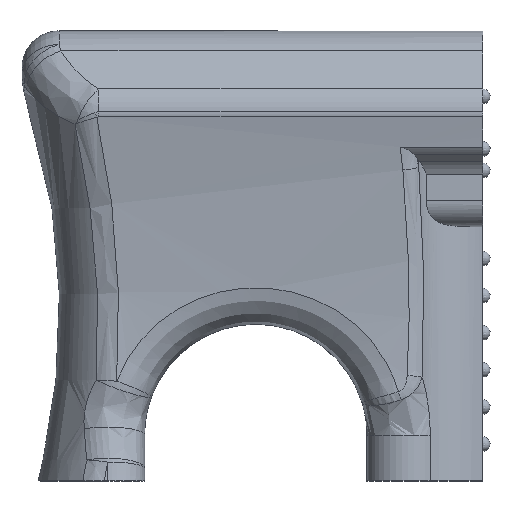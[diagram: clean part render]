
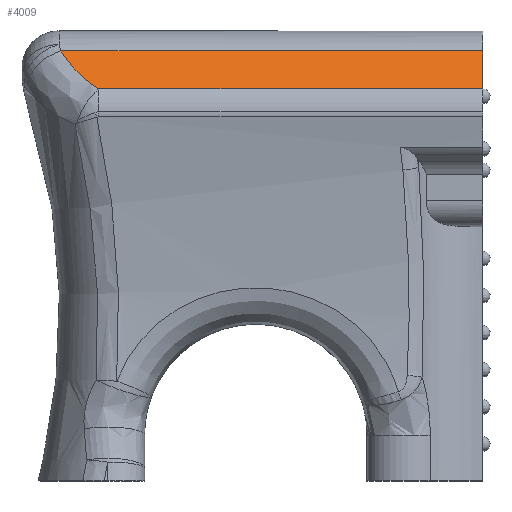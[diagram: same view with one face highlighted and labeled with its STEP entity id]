
A CAD part, top view. The second image highlights one B-rep face of the part: STEP entity #4009.
In plain terms, the highlighted planar face has unit normal (0, 0.707, 0.707).
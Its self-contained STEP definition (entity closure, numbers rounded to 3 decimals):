
#13 = VERTEX_POINT ( 'NONE', #1713 ) ;
#22 = VERTEX_POINT ( 'NONE', #1698 ) ;
#110 = CARTESIAN_POINT ( 'NONE',  ( -410.035, 72.83, 27.888 ) ) ;
#294 = CARTESIAN_POINT ( 'NONE',  ( -311.087, 82.064, 18.653 ) ) ;
#381 = LINE ( 'NONE', #110, #1824 ) ;
#393 = DIRECTION ( 'NONE',  ( 0., -0.707, 0.707 ) ) ;
#504 = EDGE_CURVE ( 'NONE', #13, #22, #2383, .T. ) ;
#752 = ORIENTED_EDGE ( 'NONE', *, *, #504, .F. ) ;
#764 = ORIENTED_EDGE ( 'NONE', *, *, #1978, .T. ) ;
#769 = FACE_OUTER_BOUND ( 'NONE', #2669, .T. ) ;
#953 = ORIENTED_EDGE ( 'NONE', *, *, #3705, .T. ) ;
#1006 = ORIENTED_EDGE ( 'NONE', *, *, #5171, .T. ) ;
#1143 = CARTESIAN_POINT ( 'NONE',  ( -310.44, 81.118, 19.6 ) ) ;
#1258 = LINE ( 'NONE', #4623, #1267 ) ;
#1267 = VECTOR ( 'NONE', #2210, 1000. ) ;
#1358 = DIRECTION ( 'NONE',  ( 0., -0.707, 0.707 ) ) ;
#1555 = CARTESIAN_POINT ( 'NONE',  ( -308.262, 78.388, 22.329 ) ) ;
#1640 = PLANE ( 'NONE',  #3135 ) ;
#1698 = CARTESIAN_POINT ( 'NONE',  ( -197.877, 72.83, 27.888 ) ) ;
#1713 = CARTESIAN_POINT ( 'NONE',  ( -197.877, 83.036, 17.682 ) ) ;
#1809 = CARTESIAN_POINT ( 'NONE',  ( -197.877, 83.036, 17.682 ) ) ;
#1824 = VECTOR ( 'NONE', #3069, 1000. ) ;
#1978 = EDGE_CURVE ( 'NONE', #13, #2704, #1258, .T. ) ;
#1986 = CARTESIAN_POINT ( 'NONE',  ( -305.692, 75.841, 24.876 ) ) ;
#2210 = DIRECTION ( 'NONE',  ( -1., 0., 0. ) ) ;
#2383 = LINE ( 'NONE', #1809, #4109 ) ;
#2404 = CARTESIAN_POINT ( 'NONE',  ( -302.64, 73.512, 27.205 ) ) ;
#2659 = VERTEX_POINT ( 'NONE', #4454 ) ;
#2669 = EDGE_LOOP ( 'NONE', ( #752, #764, #953, #1006 ) ) ;
#2704 = VERTEX_POINT ( 'NONE', #3294 ) ;
#2815 = CARTESIAN_POINT ( 'NONE',  ( -311.682, 83.036, 17.682 ) ) ;
#2913 = DIRECTION ( 'NONE',  ( 0., 0.707, 0.707 ) ) ;
#3069 = DIRECTION ( 'NONE',  ( 1., 0., 0. ) ) ;
#3135 = AXIS2_PLACEMENT_3D ( 'NONE', #5234, #2913, #393 ) ;
#3294 = CARTESIAN_POINT ( 'NONE',  ( -311.682, 83.036, 17.682 ) ) ;
#3555 = B_SPLINE_CURVE_WITH_KNOTS ( 'NONE', 3,
 ( #2815, #294, #1143, #4049, #1555, #4429, #1986, #4796, #2404, #5161 ),
 .UNSPECIFIED., .F., .F.,
 ( 4, 2, 2, 2, 4 ),
 ( 0., 0.004, 0.009, 0.013, 0.018 ),
 .UNSPECIFIED. ) ;
#3705 = EDGE_CURVE ( 'NONE', #2704, #2659, #3555, .T. ) ;
#4009 = ADVANCED_FACE ( 'NONE', ( #769 ), #1640, .T. ) ;
#4049 = CARTESIAN_POINT ( 'NONE',  ( -309.027, 79.28, 21.438 ) ) ;
#4109 = VECTOR ( 'NONE', #1358, 1000. ) ;
#4429 = CARTESIAN_POINT ( 'NONE',  ( -306.594, 76.669, 24.048 ) ) ;
#4454 = CARTESIAN_POINT ( 'NONE',  ( -301.482, 72.83, 27.888 ) ) ;
#4623 = CARTESIAN_POINT ( 'NONE',  ( -410.035, 83.036, 17.682 ) ) ;
#4796 = CARTESIAN_POINT ( 'NONE',  ( -303.718, 74.265, 26.453 ) ) ;
#5161 = CARTESIAN_POINT ( 'NONE',  ( -301.482, 72.83, 27.888 ) ) ;
#5171 = EDGE_CURVE ( 'NONE', #2659, #22, #381, .T. ) ;
#5234 = CARTESIAN_POINT ( 'NONE',  ( -410.035, 83.036, 17.682 ) ) ;
